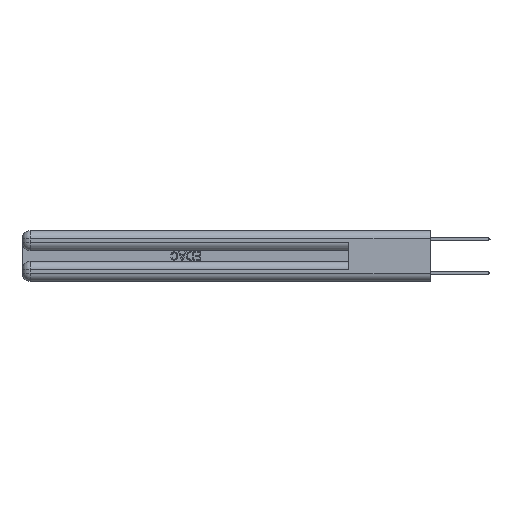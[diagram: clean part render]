
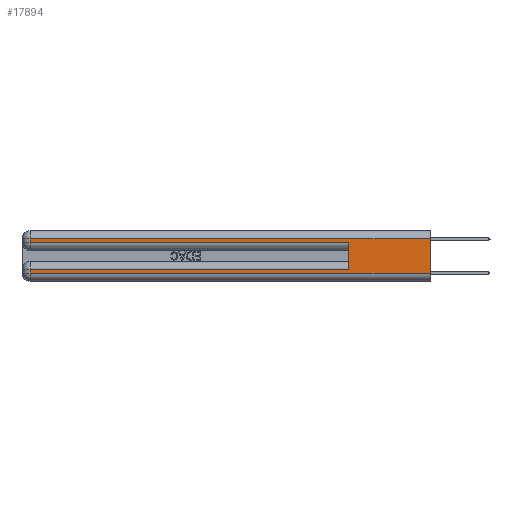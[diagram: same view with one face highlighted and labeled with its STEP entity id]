
A CAD part, left-side view. The second image highlights one B-rep face of the part: STEP entity #17894.
In plain terms, the highlighted planar face has unit normal (-1, 0, 0).
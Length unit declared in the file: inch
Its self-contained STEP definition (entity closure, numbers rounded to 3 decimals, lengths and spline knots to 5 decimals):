
#336 = AXIS2_PLACEMENT_3D ( 'NONE', #24796, #10316, #22147 ) ;
#591 = DIRECTION ( 'NONE',  ( 0., -1., 0. ) ) ;
#598 = VERTEX_POINT ( 'NONE', #13845 ) ;
#618 = CARTESIAN_POINT ( 'NONE',  ( 0., 0., 0.31 ) ) ;
#1058 = EDGE_LOOP ( 'NONE', ( #29668, #11976, #8116, #10549, #3493, #23064, #26853, #12006 ) ) ;
#1263 = CARTESIAN_POINT ( 'NONE',  ( 0., 2.94, 0.37 ) ) ;
#1939 = VERTEX_POINT ( 'NONE', #20326 ) ;
#2340 = LINE ( 'NONE', #22541, #7607 ) ;
#2384 = CARTESIAN_POINT ( 'NONE',  ( 0., 0., 0.06 ) ) ;
#2915 = VECTOR ( 'NONE', #6391, 39.37008 ) ;
#3493 = ORIENTED_EDGE ( 'NONE', *, *, #21944, .F. ) ;
#4521 = VERTEX_POINT ( 'NONE', #15794 ) ;
#4531 = VECTOR ( 'NONE', #5468, 39.37008 ) ;
#4824 = VECTOR ( 'NONE', #24387, 39.37008 ) ;
#5468 = DIRECTION ( 'NONE',  ( 0., 0., -1. ) ) ;
#5869 = LINE ( 'NONE', #618, #31756 ) ;
#6391 = DIRECTION ( 'NONE',  ( 0., 1., 0. ) ) ;
#6887 = VERTEX_POINT ( 'NONE', #22449 ) ;
#6911 = EDGE_CURVE ( 'NONE', #11378, #6887, #30524, .T. ) ;
#7607 = VECTOR ( 'NONE', #591, 39.37008 ) ;
#8116 = ORIENTED_EDGE ( 'NONE', *, *, #6911, .T. ) ;
#8212 = DIRECTION ( 'NONE',  ( 0., 0., -1. ) ) ;
#10316 = DIRECTION ( 'NONE',  ( 1., 0., 0. ) ) ;
#10549 = ORIENTED_EDGE ( 'NONE', *, *, #15930, .T. ) ;
#10687 = VERTEX_POINT ( 'NONE', #27056 ) ;
#11378 = VERTEX_POINT ( 'NONE', #32940 ) ;
#11976 = ORIENTED_EDGE ( 'NONE', *, *, #32718, .T. ) ;
#12006 = ORIENTED_EDGE ( 'NONE', *, *, #14293, .T. ) ;
#12068 = DIRECTION ( 'NONE',  ( 0., 1., 0. ) ) ;
#12538 = EDGE_CURVE ( 'NONE', #10687, #28875, #34482, .T. ) ;
#13845 = CARTESIAN_POINT ( 'NONE',  ( 0., 0., 0.31 ) ) ;
#14293 = EDGE_CURVE ( 'NONE', #4521, #22481, #2340, .T. ) ;
#15794 = CARTESIAN_POINT ( 'NONE',  ( 0., 2.94, 0.06 ) ) ;
#15930 = EDGE_CURVE ( 'NONE', #6887, #1939, #20041, .T. ) ;
#16581 = PLANE ( 'NONE',  #336 ) ;
#17894 = ADVANCED_FACE ( 'NONE', ( #18167 ), #16581, .F. ) ;
#18167 = FACE_OUTER_BOUND ( 'NONE', #1058, .T. ) ;
#18843 = CARTESIAN_POINT ( 'NONE',  ( 0., 0.6, 0.145 ) ) ;
#19186 = LINE ( 'NONE', #18843, #29482 ) ;
#19608 = CARTESIAN_POINT ( 'NONE',  ( 0., 0., 0.37 ) ) ;
#19978 = CARTESIAN_POINT ( 'NONE',  ( 0., 0., 0.085 ) ) ;
#20041 = LINE ( 'NONE', #32527, #4824 ) ;
#20138 = LINE ( 'NONE', #19608, #33851 ) ;
#20326 = CARTESIAN_POINT ( 'NONE',  ( 0., 0.6, 0.285 ) ) ;
#20412 = EDGE_CURVE ( 'NONE', #28875, #4521, #22303, .T. ) ;
#21501 = DIRECTION ( 'NONE',  ( 0., 0., 1. ) ) ;
#21944 = EDGE_CURVE ( 'NONE', #10687, #1939, #19186, .T. ) ;
#22147 = DIRECTION ( 'NONE',  ( 0., 0., -1. ) ) ;
#22303 = LINE ( 'NONE', #1263, #4531 ) ;
#22449 = CARTESIAN_POINT ( 'NONE',  ( 0., 2.94, 0.285 ) ) ;
#22481 = VERTEX_POINT ( 'NONE', #2384 ) ;
#22541 = CARTESIAN_POINT ( 'NONE',  ( 0., 0., 0.06 ) ) ;
#22588 = CARTESIAN_POINT ( 'NONE',  ( 0., 2.94, 0.085 ) ) ;
#23064 = ORIENTED_EDGE ( 'NONE', *, *, #12538, .T. ) ;
#23273 = VECTOR ( 'NONE', #8212, 39.37008 ) ;
#24387 = DIRECTION ( 'NONE',  ( 0., -1., 0. ) ) ;
#24796 = CARTESIAN_POINT ( 'NONE',  ( 0., 0., 0.37 ) ) ;
#26853 = ORIENTED_EDGE ( 'NONE', *, *, #20412, .T. ) ;
#27056 = CARTESIAN_POINT ( 'NONE',  ( 0., 0.6, 0.085 ) ) ;
#27768 = DIRECTION ( 'NONE',  ( 0., 0., -1. ) ) ;
#27821 = CARTESIAN_POINT ( 'NONE',  ( 0., 2.94, 0.37 ) ) ;
#28875 = VERTEX_POINT ( 'NONE', #22588 ) ;
#29482 = VECTOR ( 'NONE', #21501, 39.37008 ) ;
#29668 = ORIENTED_EDGE ( 'NONE', *, *, #33727, .F. ) ;
#30524 = LINE ( 'NONE', #27821, #23273 ) ;
#31756 = VECTOR ( 'NONE', #12068, 39.37008 ) ;
#32527 = CARTESIAN_POINT ( 'NONE',  ( 0., 0., 0.285 ) ) ;
#32718 = EDGE_CURVE ( 'NONE', #598, #11378, #5869, .T. ) ;
#32940 = CARTESIAN_POINT ( 'NONE',  ( 0., 2.94, 0.31 ) ) ;
#33727 = EDGE_CURVE ( 'NONE', #598, #22481, #20138, .T. ) ;
#33851 = VECTOR ( 'NONE', #27768, 39.37008 ) ;
#34482 = LINE ( 'NONE', #19978, #2915 ) ;
